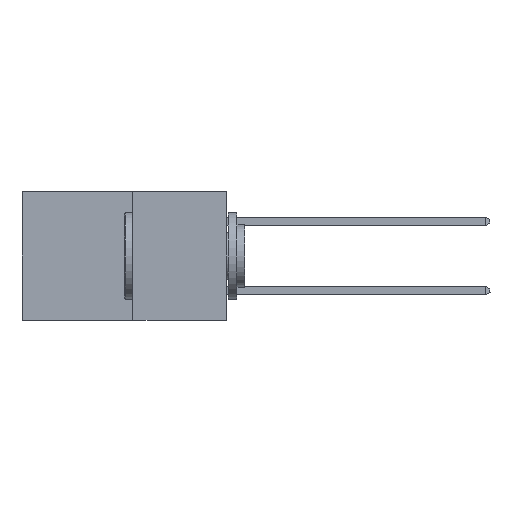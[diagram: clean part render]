
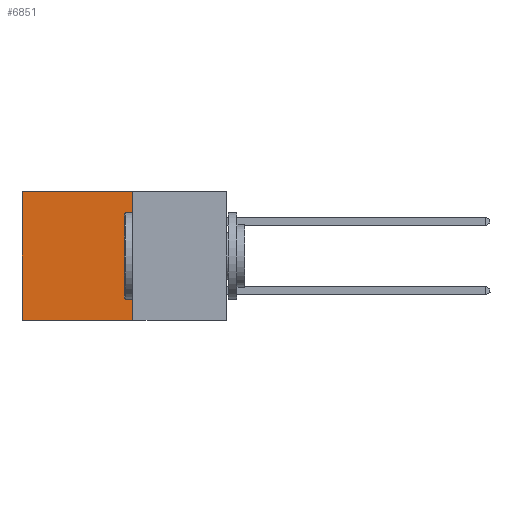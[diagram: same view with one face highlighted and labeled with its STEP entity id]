
A CAD part, left-side view. The second image highlights one B-rep face of the part: STEP entity #6851.
In plain terms, the highlighted planar face has unit normal (-1, 0, 0).
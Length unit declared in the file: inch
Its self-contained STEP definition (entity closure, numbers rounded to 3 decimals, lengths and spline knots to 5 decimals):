
#882 = EDGE_CURVE ( 'NONE', #7802, #8497, #1255, .T. ) ;
#992 = ORIENTED_EDGE ( 'NONE', *, *, #6652, .T. ) ;
#1141 = ORIENTED_EDGE ( 'NONE', *, *, #3879, .F. ) ;
#1200 = DIRECTION ( 'NONE',  ( 1., 0., 0. ) ) ;
#1255 = LINE ( 'NONE', #2552, #3589 ) ;
#1441 = VERTEX_POINT ( 'NONE', #7965 ) ;
#1537 = ORIENTED_EDGE ( 'NONE', *, *, #882, .F. ) ;
#1540 = LINE ( 'NONE', #4333, #8408 ) ;
#1923 = ORIENTED_EDGE ( 'NONE', *, *, #3313, .T. ) ;
#2552 = CARTESIAN_POINT ( 'NONE',  ( 0.277, 0.27, -0.37 ) ) ;
#2717 = CARTESIAN_POINT ( 'NONE',  ( 0.277, 0.27, -0.37 ) ) ;
#2892 = EDGE_LOOP ( 'NONE', ( #992, #1141, #1537, #1923 ) ) ;
#3313 = EDGE_CURVE ( 'NONE', #7802, #1441, #1540, .T. ) ;
#3492 = FACE_OUTER_BOUND ( 'NONE', #2892, .T. ) ;
#3589 = VECTOR ( 'NONE', #7586, 39.37008 ) ;
#3654 = CARTESIAN_POINT ( 'NONE',  ( 0.277, 0.27, -0.37 ) ) ;
#3879 = EDGE_CURVE ( 'NONE', #8497, #5082, #7241, .T. ) ;
#4267 = VECTOR ( 'NONE', #8379, 39.37008 ) ;
#4333 = CARTESIAN_POINT ( 'NONE',  ( 0.277, 0.27, 0. ) ) ;
#4352 = DIRECTION ( 'NONE',  ( 0., 1., 0. ) ) ;
#4642 = PLANE ( 'NONE',  #8046 ) ;
#4945 = LINE ( 'NONE', #7608, #8045 ) ;
#5082 = VERTEX_POINT ( 'NONE', #7974 ) ;
#5311 = CARTESIAN_POINT ( 'NONE',  ( 0.277, 0.27, -0.37 ) ) ;
#5560 = CARTESIAN_POINT ( 'NONE',  ( 0.277, 0.27, 0. ) ) ;
#5962 = DIRECTION ( 'NONE',  ( 0., 0., -1. ) ) ;
#6652 = EDGE_CURVE ( 'NONE', #1441, #5082, #4945, .T. ) ;
#6851 = ADVANCED_FACE ( 'NONE', ( #3492 ), #4642, .F. ) ;
#7011 = DIRECTION ( 'NONE',  ( 0., 0., -1. ) ) ;
#7241 = LINE ( 'NONE', #2717, #4267 ) ;
#7586 = DIRECTION ( 'NONE',  ( 0., 0., -1. ) ) ;
#7608 = CARTESIAN_POINT ( 'NONE',  ( 0.277, 0.59, -0.37 ) ) ;
#7802 = VERTEX_POINT ( 'NONE', #5560 ) ;
#7965 = CARTESIAN_POINT ( 'NONE',  ( 0.277, 0.59, 0. ) ) ;
#7974 = CARTESIAN_POINT ( 'NONE',  ( 0.277, 0.59, -0.37 ) ) ;
#8045 = VECTOR ( 'NONE', #7011, 39.37008 ) ;
#8046 = AXIS2_PLACEMENT_3D ( 'NONE', #5311, #1200, #5962 ) ;
#8379 = DIRECTION ( 'NONE',  ( 0., 1., 0. ) ) ;
#8408 = VECTOR ( 'NONE', #4352, 39.37008 ) ;
#8497 = VERTEX_POINT ( 'NONE', #3654 ) ;
